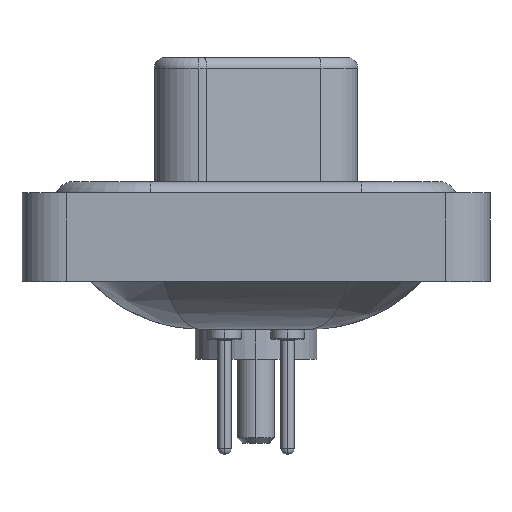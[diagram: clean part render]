
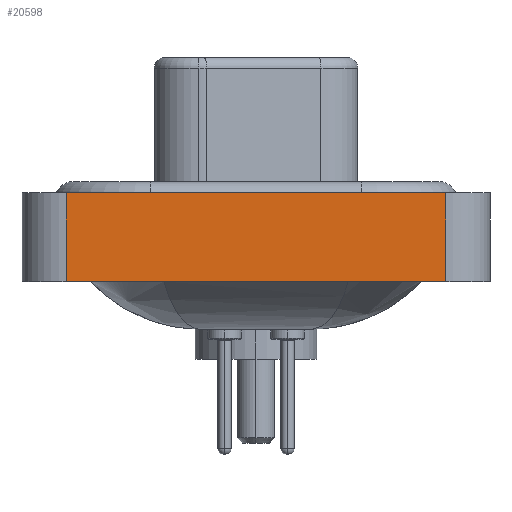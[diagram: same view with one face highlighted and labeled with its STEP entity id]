
A CAD part, left-side view. The second image highlights one B-rep face of the part: STEP entity #20598.
In plain terms, the highlighted planar face has unit normal (-1, 0, 0).
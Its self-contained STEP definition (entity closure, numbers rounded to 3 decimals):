
#264 = CARTESIAN_POINT ( 'NONE',  ( -7.3, -8.55, 0.4 ) ) ;
#966 = AXIS2_PLACEMENT_3D ( 'NONE', #6905, #15163, #18198 ) ;
#3294 = CARTESIAN_POINT ( 'NONE',  ( -7.3, -8.55, -3.6 ) ) ;
#3308 = LINE ( 'NONE', #20344, #17338 ) ;
#3831 = EDGE_CURVE ( 'NONE', #13063, #12830, #15855, .T. ) ;
#4354 = DIRECTION ( 'NONE',  ( 0., 0., 1. ) ) ;
#6026 = VECTOR ( 'NONE', #12593, 1000. ) ;
#6031 = DIRECTION ( 'NONE',  ( 0., -1., 0. ) ) ;
#6111 = LINE ( 'NONE', #17201, #6026 ) ;
#6622 = ORIENTED_EDGE ( 'NONE', *, *, #16709, .F. ) ;
#6905 = CARTESIAN_POINT ( 'NONE',  ( -7.3, -8.55, -3.6 ) ) ;
#6910 = VERTEX_POINT ( 'NONE', #264 ) ;
#6977 = EDGE_CURVE ( 'NONE', #13427, #6910, #7905, .T. ) ;
#7758 = CARTESIAN_POINT ( 'NONE',  ( -7.3, 8.55, 0.4 ) ) ;
#7905 = LINE ( 'NONE', #3294, #10903 ) ;
#8453 = EDGE_LOOP ( 'NONE', ( #14748, #6622, #12142, #10727 ) ) ;
#10727 = ORIENTED_EDGE ( 'NONE', *, *, #18037, .T. ) ;
#10903 = VECTOR ( 'NONE', #14289, 1000. ) ;
#12142 = ORIENTED_EDGE ( 'NONE', *, *, #3831, .F. ) ;
#12304 = CARTESIAN_POINT ( 'NONE',  ( -7.3, 8.55, -3.6 ) ) ;
#12593 = DIRECTION ( 'NONE',  ( 0., -1., 0. ) ) ;
#12830 = VERTEX_POINT ( 'NONE', #7758 ) ;
#13063 = VERTEX_POINT ( 'NONE', #13068 ) ;
#13068 = CARTESIAN_POINT ( 'NONE',  ( -7.3, 8.55, -3.6 ) ) ;
#13427 = VERTEX_POINT ( 'NONE', #16287 ) ;
#14289 = DIRECTION ( 'NONE',  ( 0., 0., 1. ) ) ;
#14748 = ORIENTED_EDGE ( 'NONE', *, *, #6977, .T. ) ;
#15057 = PLANE ( 'NONE',  #966 ) ;
#15163 = DIRECTION ( 'NONE',  ( -1., 0., 0. ) ) ;
#15855 = LINE ( 'NONE', #12304, #18809 ) ;
#16287 = CARTESIAN_POINT ( 'NONE',  ( -7.3, -8.55, -3.6 ) ) ;
#16709 = EDGE_CURVE ( 'NONE', #12830, #6910, #3308, .T. ) ;
#17201 = CARTESIAN_POINT ( 'NONE',  ( -7.3, -8.55, -3.6 ) ) ;
#17338 = VECTOR ( 'NONE', #6031, 1000. ) ;
#18037 = EDGE_CURVE ( 'NONE', #13063, #13427, #6111, .T. ) ;
#18198 = DIRECTION ( 'NONE',  ( 0., 0., 1. ) ) ;
#18809 = VECTOR ( 'NONE', #4354, 1000. ) ;
#20059 = FACE_OUTER_BOUND ( 'NONE', #8453, .T. ) ;
#20344 = CARTESIAN_POINT ( 'NONE',  ( -7.3, -8.55, 0.4 ) ) ;
#20598 = ADVANCED_FACE ( 'NONE', ( #20059 ), #15057, .T. ) ;
